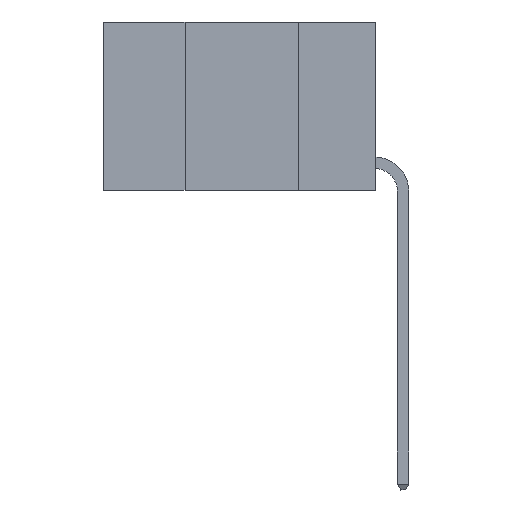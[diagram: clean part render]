
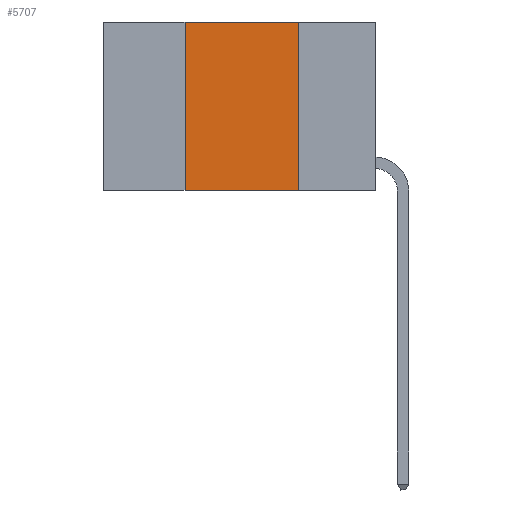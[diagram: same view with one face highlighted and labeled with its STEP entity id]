
A CAD part, left-side view. The second image highlights one B-rep face of the part: STEP entity #5707.
In plain terms, the highlighted planar face has unit normal (-1, 0, 0).
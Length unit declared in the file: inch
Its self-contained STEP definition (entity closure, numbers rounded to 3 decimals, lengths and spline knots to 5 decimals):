
#138 = VECTOR ( 'NONE', #13624, 39.37008 ) ;
#558 = PLANE ( 'NONE',  #6538 ) ;
#1076 = CARTESIAN_POINT ( 'NONE',  ( 0., 0.17, 0. ) ) ;
#1151 = VECTOR ( 'NONE', #9911, 39.37008 ) ;
#1158 = ORIENTED_EDGE ( 'NONE', *, *, #11678, .F. ) ;
#1440 = ORIENTED_EDGE ( 'NONE', *, *, #13638, .F. ) ;
#1708 = FACE_OUTER_BOUND ( 'NONE', #13602, .T. ) ;
#1908 = VERTEX_POINT ( 'NONE', #5005 ) ;
#1971 = CARTESIAN_POINT ( 'NONE',  ( 0., 0.42, -0.37 ) ) ;
#2032 = VERTEX_POINT ( 'NONE', #1076 ) ;
#3387 = LINE ( 'NONE', #9292, #13348 ) ;
#3447 = DIRECTION ( 'NONE',  ( 0., 0., -1. ) ) ;
#5005 = CARTESIAN_POINT ( 'NONE',  ( 0., 0.42, 0. ) ) ;
#5258 = VERTEX_POINT ( 'NONE', #8809 ) ;
#5707 = ADVANCED_FACE ( 'NONE', ( #1708 ), #558, .F. ) ;
#6370 = EDGE_CURVE ( 'NONE', #1908, #2032, #3387, .T. ) ;
#6493 = DIRECTION ( 'NONE',  ( 1., 0., 0. ) ) ;
#6538 = AXIS2_PLACEMENT_3D ( 'NONE', #15095, #6493, #7762 ) ;
#6992 = CARTESIAN_POINT ( 'NONE',  ( 0., 0.17, 0. ) ) ;
#7762 = DIRECTION ( 'NONE',  ( 0., 0., -1. ) ) ;
#8598 = CARTESIAN_POINT ( 'NONE',  ( 0., 0.42, 0. ) ) ;
#8809 = CARTESIAN_POINT ( 'NONE',  ( 0., 0.17, -0.37 ) ) ;
#8822 = LINE ( 'NONE', #8598, #138 ) ;
#9292 = CARTESIAN_POINT ( 'NONE',  ( 0., 0.6, 0. ) ) ;
#9911 = DIRECTION ( 'NONE',  ( 0., -1., 0. ) ) ;
#10067 = EDGE_CURVE ( 'NONE', #11837, #5258, #13878, .T. ) ;
#10479 = VECTOR ( 'NONE', #3447, 39.37008 ) ;
#10919 = ORIENTED_EDGE ( 'NONE', *, *, #10067, .T. ) ;
#11320 = LINE ( 'NONE', #6992, #10479 ) ;
#11678 = EDGE_CURVE ( 'NONE', #11837, #1908, #8822, .T. ) ;
#11837 = VERTEX_POINT ( 'NONE', #1971 ) ;
#12464 = ORIENTED_EDGE ( 'NONE', *, *, #6370, .F. ) ;
#13348 = VECTOR ( 'NONE', #13950, 39.37008 ) ;
#13602 = EDGE_LOOP ( 'NONE', ( #1440, #12464, #1158, #10919 ) ) ;
#13624 = DIRECTION ( 'NONE',  ( 0., 0., 1. ) ) ;
#13638 = EDGE_CURVE ( 'NONE', #2032, #5258, #11320, .T. ) ;
#13718 = CARTESIAN_POINT ( 'NONE',  ( 0., 0.6, -0.37 ) ) ;
#13878 = LINE ( 'NONE', #13718, #1151 ) ;
#13950 = DIRECTION ( 'NONE',  ( 0., -1., 0. ) ) ;
#15095 = CARTESIAN_POINT ( 'NONE',  ( 0., 0.6, 0. ) ) ;
